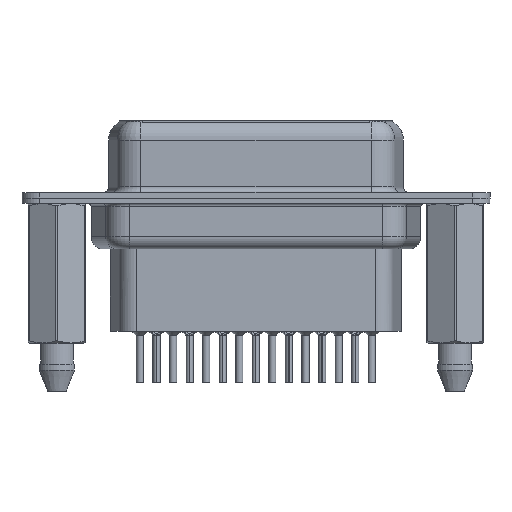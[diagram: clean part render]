
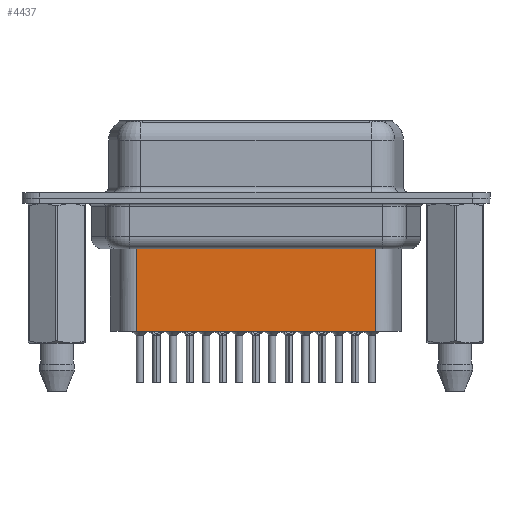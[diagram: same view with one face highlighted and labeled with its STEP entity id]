
A CAD part, front view. The second image highlights one B-rep face of the part: STEP entity #4437.
In plain terms, the highlighted planar face has unit normal (0, -1, 0).
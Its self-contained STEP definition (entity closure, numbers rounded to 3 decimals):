
#350 = EDGE_CURVE ( 'NONE', #821, #5457, #10256, .T. ) ;
#821 = VERTEX_POINT ( 'NONE', #19840 ) ;
#3735 = ORIENTED_EDGE ( 'NONE', *, *, #12469, .T. ) ;
#4270 = DIRECTION ( 'NONE',  ( -1., 0., 0. ) ) ;
#4437 = ADVANCED_FACE ( 'NONE', ( #16495 ), #24249, .T. ) ;
#4930 = VECTOR ( 'NONE', #22095, 1000. ) ;
#4950 = DIRECTION ( 'NONE',  ( 0., -1., 0. ) ) ;
#5221 = VERTEX_POINT ( 'NONE', #10613 ) ;
#5457 = VERTEX_POINT ( 'NONE', #5877 ) ;
#5766 = EDGE_CURVE ( 'NONE', #15660, #5457, #14756, .T. ) ;
#5877 = CARTESIAN_POINT ( 'NONE',  ( 6.681, -3.5, -11.15 ) ) ;
#6296 = CARTESIAN_POINT ( 'NONE',  ( 26.619, -3.5, -3.1 ) ) ;
#6620 = CARTESIAN_POINT ( 'NONE',  ( 6.434, -3.5, -4.097 ) ) ;
#6861 = DIRECTION ( 'NONE',  ( 1., 0., 0. ) ) ;
#7267 = CARTESIAN_POINT ( 'NONE',  ( 6.681, -3.5, -3.1 ) ) ;
#8468 = CARTESIAN_POINT ( 'NONE',  ( 6.681, -3.5, -11.15 ) ) ;
#9168 = EDGE_CURVE ( 'NONE', #5221, #821, #9998, .T. ) ;
#9222 = AXIS2_PLACEMENT_3D ( 'NONE', #14724, #4950, #6861 ) ;
#9998 = LINE ( 'NONE', #6296, #17423 ) ;
#10256 = LINE ( 'NONE', #8468, #13918 ) ;
#10393 = ORIENTED_EDGE ( 'NONE', *, *, #350, .F. ) ;
#10489 = ORIENTED_EDGE ( 'NONE', *, *, #9168, .F. ) ;
#10613 = CARTESIAN_POINT ( 'NONE',  ( 26.619, -3.5, -4.097 ) ) ;
#12386 = DIRECTION ( 'NONE',  ( 0., 0., -1. ) ) ;
#12469 = EDGE_CURVE ( 'NONE', #5221, #15660, #14354, .T. ) ;
#12994 = DIRECTION ( 'NONE',  ( 0., 0., -1. ) ) ;
#13391 = EDGE_LOOP ( 'NONE', ( #10489, #3735, #24361, #10393 ) ) ;
#13918 = VECTOR ( 'NONE', #4270, 1000. ) ;
#14354 = LINE ( 'NONE', #6620, #4930 ) ;
#14724 = CARTESIAN_POINT ( 'NONE',  ( 6.681, -3.5, -3.1 ) ) ;
#14756 = LINE ( 'NONE', #7267, #17299 ) ;
#15660 = VERTEX_POINT ( 'NONE', #21133 ) ;
#16495 = FACE_OUTER_BOUND ( 'NONE', #13391, .T. ) ;
#17299 = VECTOR ( 'NONE', #12994, 1000. ) ;
#17423 = VECTOR ( 'NONE', #12386, 1000. ) ;
#19840 = CARTESIAN_POINT ( 'NONE',  ( 26.619, -3.5, -11.15 ) ) ;
#21133 = CARTESIAN_POINT ( 'NONE',  ( 6.681, -3.5, -4.097 ) ) ;
#22095 = DIRECTION ( 'NONE',  ( -1., 0., 0. ) ) ;
#24249 = PLANE ( 'NONE',  #9222 ) ;
#24361 = ORIENTED_EDGE ( 'NONE', *, *, #5766, .T. ) ;
